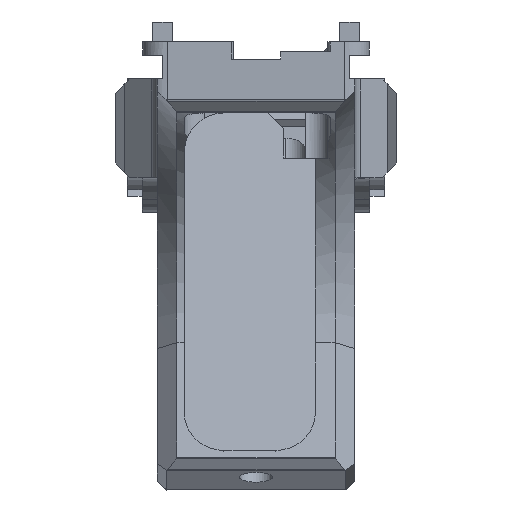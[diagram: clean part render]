
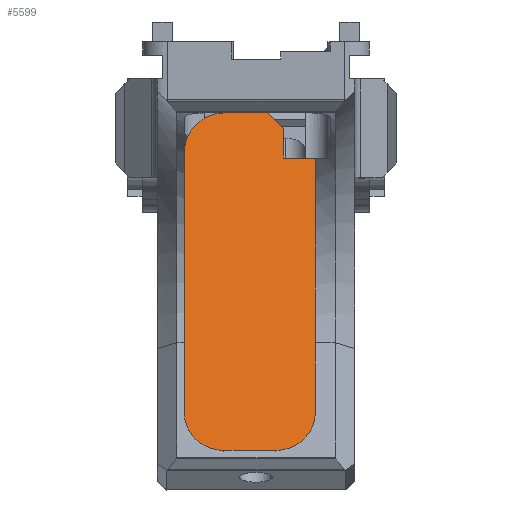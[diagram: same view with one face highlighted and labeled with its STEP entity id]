
A CAD part, left-side view. The second image highlights one B-rep face of the part: STEP entity #5599.
In plain terms, the highlighted planar face has unit normal (-0.956, 0, 0.292).
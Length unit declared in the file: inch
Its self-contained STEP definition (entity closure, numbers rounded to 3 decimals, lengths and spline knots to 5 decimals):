
#213=CIRCLE('',#5989,0.15748);
#222=CIRCLE('',#6018,0.15748);
#529=FACE_OUTER_BOUND('',#825,.T.);
#825=EDGE_LOOP('',(#4548,#4549,#4550,#4551,#4552,#4553,#4554,#4555,#4556,
#4557,#4558));
#1007=LINE('',#8108,#1616);
#1293=LINE('',#8954,#1902);
#1295=LINE('',#8961,#1904);
#1364=LINE('',#9186,#1973);
#1366=LINE('',#9189,#1975);
#1373=LINE('',#9204,#1982);
#1374=LINE('',#9205,#1983);
#1375=LINE('',#9206,#1984);
#1376=LINE('',#9207,#1985);
#1616=VECTOR('',#6411,1.);
#1902=VECTOR('',#7081,1.);
#1904=VECTOR('',#7091,1.);
#1973=VECTOR('',#7278,1.);
#1975=VECTOR('',#7282,1.);
#1982=VECTOR('',#7299,1.);
#1983=VECTOR('',#7300,1.);
#1984=VECTOR('',#7301,1.);
#1985=VECTOR('',#7302,1.);
#2243=VERTEX_POINT('',#8105);
#2244=VERTEX_POINT('',#8107);
#2534=VERTEX_POINT('',#8951);
#2535=VERTEX_POINT('',#8953);
#2536=VERTEX_POINT('',#8960);
#2547=VERTEX_POINT('',#8991);
#2564=VERTEX_POINT('',#9048);
#2596=VERTEX_POINT('',#9183);
#2597=VERTEX_POINT('',#9185);
#2599=VERTEX_POINT('',#9202);
#2600=VERTEX_POINT('',#9203);
#2818=EDGE_CURVE('',#2244,#2243,#1007,.T.);
#3206=EDGE_CURVE('',#2535,#2534,#1293,.T.);
#3209=EDGE_CURVE('',#2243,#2535,#213,.T.);
#3210=EDGE_CURVE('',#2536,#2244,#1295,.T.);
#3254=EDGE_CURVE('',#2534,#2564,#222,.T.);
#3307=EDGE_CURVE('',#2596,#2597,#1364,.T.);
#3309=EDGE_CURVE('',#2536,#2596,#1366,.T.);
#3317=EDGE_CURVE('',#2599,#2600,#1373,.T.);
#3318=EDGE_CURVE('',#2600,#2597,#1374,.T.);
#3319=EDGE_CURVE('',#2547,#2564,#1375,.T.);
#3320=EDGE_CURVE('',#2599,#2547,#1376,.T.);
#4548=ORIENTED_EDGE('',*,*,#3317,.T.);
#4549=ORIENTED_EDGE('',*,*,#3318,.T.);
#4550=ORIENTED_EDGE('',*,*,#3307,.F.);
#4551=ORIENTED_EDGE('',*,*,#3309,.F.);
#4552=ORIENTED_EDGE('',*,*,#3210,.T.);
#4553=ORIENTED_EDGE('',*,*,#2818,.T.);
#4554=ORIENTED_EDGE('',*,*,#3209,.T.);
#4555=ORIENTED_EDGE('',*,*,#3206,.T.);
#4556=ORIENTED_EDGE('',*,*,#3254,.T.);
#4557=ORIENTED_EDGE('',*,*,#3319,.F.);
#4558=ORIENTED_EDGE('',*,*,#3320,.F.);
#5358=PLANE('',#6055);
#5599=ADVANCED_FACE('',(#529),#5358,.F.);
#5989=AXIS2_PLACEMENT_3D('',#8958,#7087,#7088);
#6018=AXIS2_PLACEMENT_3D('',#9049,#7178,#7179);
#6055=AXIS2_PLACEMENT_3D('',#9201,#7297,#7298);
#6411=DIRECTION('',(-0.292,0.,-0.956));
#7081=DIRECTION('',(0.,-1.,0.));
#7087=DIRECTION('center_axis',(-0.956,0.,0.292));
#7088=DIRECTION('ref_axis',(-0.207,0.707,-0.676));
#7091=DIRECTION('',(-0.292,0.,-0.956));
#7178=DIRECTION('center_axis',(-0.956,0.,
0.292));
#7179=DIRECTION('ref_axis',(-0.207,-0.707,-0.676));
#7278=DIRECTION('',(-0.211,-0.691,-0.691));
#7282=DIRECTION('',(0.,-1.,0.));
#7297=DIRECTION('center_axis',(0.956,0.,-0.292));
#7298=DIRECTION('ref_axis',(0.,-1.,0.));
#7299=DIRECTION('',(0.,1.,0.));
#7300=DIRECTION('',(0.292,0.,0.956));
#7301=DIRECTION('',(-0.292,0.,-0.956));
#7302=DIRECTION('',(-0.292,0.,-0.956));
#8105=CARTESIAN_POINT('',(0.78518,0.28543,-1.68854));
#8107=CARTESIAN_POINT('',(1.03016,0.28543,-0.88724));
#8108=CARTESIAN_POINT('',(1.15276,0.28543,-0.48624));
#8951=CARTESIAN_POINT('',(0.73914,-0.07874,-1.83914));
#8953=CARTESIAN_POINT('',(0.73914,0.12795,-1.83914));
#8954=CARTESIAN_POINT('',(0.73914,0.08366,-1.83914));
#8958=CARTESIAN_POINT('Origin',(0.78518,0.12795,-1.68854));
#8960=CARTESIAN_POINT('',(1.21557,0.28543,-0.28079));
#8961=CARTESIAN_POINT('',(1.15276,0.28543,-0.48624));
#8991=CARTESIAN_POINT('',(1.03016,-0.23622,-0.88724));
#9048=CARTESIAN_POINT('',(0.78518,-0.23622,-1.68854));
#9049=CARTESIAN_POINT('Origin',(0.78518,-0.07874,-1.68854));
#9183=CARTESIAN_POINT('',(1.21557,0.08858,-0.28079));
#9185=CARTESIAN_POINT('',(1.15539,-0.10827,-0.47764));
#9186=CARTESIAN_POINT('',(1.18114,-0.02405,-0.39342));
#9189=CARTESIAN_POINT('',(1.21557,0.01969,-0.28079));
#9201=CARTESIAN_POINT('Origin',(1.15169,0.03937,-0.48973));
#9202=CARTESIAN_POINT('',(1.11928,-0.23622,-0.59575));
#9203=CARTESIAN_POINT('',(1.11928,-0.10827,-0.59575));
#9204=CARTESIAN_POINT('',(1.11928,-0.02531,-0.59575));
#9205=CARTESIAN_POINT('',(1.16094,-0.10827,-0.45949));
#9206=CARTESIAN_POINT('',(1.19672,-0.23622,-0.34246));
#9207=CARTESIAN_POINT('',(1.19672,-0.23622,-0.34246));
